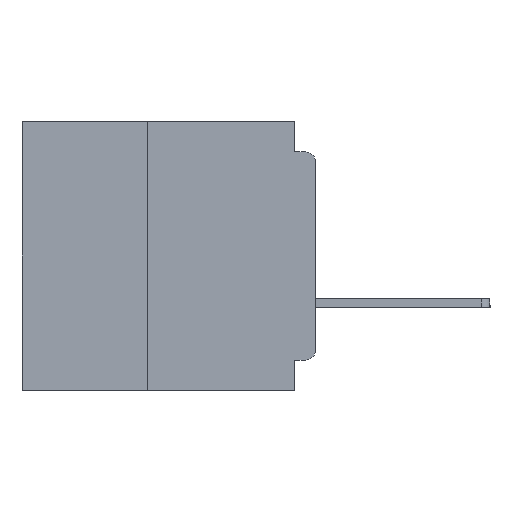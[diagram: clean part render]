
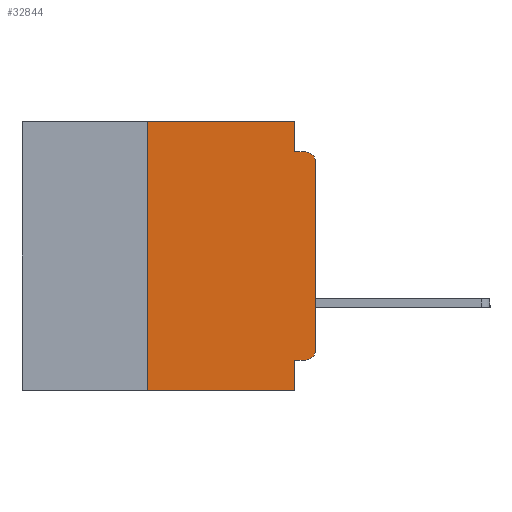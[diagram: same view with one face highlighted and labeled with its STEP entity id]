
A CAD part, left-side view. The second image highlights one B-rep face of the part: STEP entity #32844.
In plain terms, the highlighted planar face has unit normal (-1, 0, 0).
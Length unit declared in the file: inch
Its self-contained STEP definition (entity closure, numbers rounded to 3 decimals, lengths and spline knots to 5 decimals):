
#285 = CARTESIAN_POINT ( 'NONE',  ( 0., 0.031, 0. ) ) ;
#954 = VERTEX_POINT ( 'NONE', #4387 ) ;
#1689 = VERTEX_POINT ( 'NONE', #49540 ) ;
#2049 = AXIS2_PLACEMENT_3D ( 'NONE', #21257, #50289, #25529 ) ;
#2077 = VECTOR ( 'NONE', #4523, 39.37008 ) ;
#2186 = DIRECTION ( 'NONE',  ( 0., 0., 1. ) ) ;
#3131 = AXIS2_PLACEMENT_3D ( 'NONE', #6478, #35747, #10696 ) ;
#3907 = DIRECTION ( 'NONE',  ( 0., 0., 1. ) ) ;
#4387 = CARTESIAN_POINT ( 'NONE',  ( 0., 0.031, 0. ) ) ;
#4523 = DIRECTION ( 'NONE',  ( 0., 0., -1. ) ) ;
#4604 = CARTESIAN_POINT ( 'NONE',  ( 0., 0.031, -0.4 ) ) ;
#5560 = DIRECTION ( 'NONE',  ( 0., -1., 0. ) ) ;
#6478 = CARTESIAN_POINT ( 'NONE',  ( 0., 0.015, -0.06 ) ) ;
#6926 = ORIENTED_EDGE ( 'NONE', *, *, #47745, .F. ) ;
#7359 = EDGE_LOOP ( 'NONE', ( #17656, #30911, #20954, #6926, #18402, #23933, #37663, #18087, #9277, #52777 ) ) ;
#7463 = VERTEX_POINT ( 'NONE', #11105 ) ;
#7567 = DIRECTION ( 'NONE',  ( 1., 0., 0. ) ) ;
#7689 = CARTESIAN_POINT ( 'NONE',  ( 0., 0.437, 0. ) ) ;
#8110 = CARTESIAN_POINT ( 'NONE',  ( 0., 0.437, -0.4 ) ) ;
#9277 = ORIENTED_EDGE ( 'NONE', *, *, #38610, .F. ) ;
#10324 = CARTESIAN_POINT ( 'NONE',  ( 0., 0.031, -0.355 ) ) ;
#10675 = DIRECTION ( 'NONE',  ( 0., 1., 0. ) ) ;
#10696 = DIRECTION ( 'NONE',  ( 0., 0., -1. ) ) ;
#10707 = CARTESIAN_POINT ( 'NONE',  ( 0., 0.031, -0.045 ) ) ;
#11105 = CARTESIAN_POINT ( 'NONE',  ( 0., 0.015, -0.045 ) ) ;
#11180 = CARTESIAN_POINT ( 'NONE',  ( 0., 0.031, -0.4 ) ) ;
#11602 = VECTOR ( 'NONE', #5560, 39.37008 ) ;
#12342 = DIRECTION ( 'NONE',  ( 0., -1., 0. ) ) ;
#12680 = VECTOR ( 'NONE', #3907, 39.37008 ) ;
#13658 = VERTEX_POINT ( 'NONE', #24235 ) ;
#14027 = LINE ( 'NONE', #53820, #12680 ) ;
#17397 = CARTESIAN_POINT ( 'NONE',  ( 0., 0.25, -0.4 ) ) ;
#17582 = VECTOR ( 'NONE', #2186, 39.37008 ) ;
#17656 = ORIENTED_EDGE ( 'NONE', *, *, #22435, .T. ) ;
#18014 = VERTEX_POINT ( 'NONE', #10324 ) ;
#18087 = ORIENTED_EDGE ( 'NONE', *, *, #38323, .F. ) ;
#18402 = ORIENTED_EDGE ( 'NONE', *, *, #29087, .F. ) ;
#18899 = LINE ( 'NONE', #43795, #17582 ) ;
#20417 = VERTEX_POINT ( 'NONE', #11180 ) ;
#20954 = ORIENTED_EDGE ( 'NONE', *, *, #46346, .F. ) ;
#21257 = CARTESIAN_POINT ( 'NONE',  ( 0., 0.015, -0.34 ) ) ;
#21831 = EDGE_CURVE ( 'NONE', #1689, #7463, #37827, .T. ) ;
#22324 = CARTESIAN_POINT ( 'NONE',  ( 0., 0.25, 0. ) ) ;
#22435 = EDGE_CURVE ( 'NONE', #38889, #1689, #18899, .T. ) ;
#22738 = VECTOR ( 'NONE', #10675, 39.37008 ) ;
#22777 = LINE ( 'NONE', #30699, #11602 ) ;
#23933 = ORIENTED_EDGE ( 'NONE', *, *, #40884, .F. ) ;
#24235 = CARTESIAN_POINT ( 'NONE',  ( 0., 0.015, -0.355 ) ) ;
#24778 = VECTOR ( 'NONE', #12342, 39.37008 ) ;
#25529 = DIRECTION ( 'NONE',  ( 0., 0., -1. ) ) ;
#25996 = VERTEX_POINT ( 'NONE', #22324 ) ;
#26074 = VECTOR ( 'NONE', #38063, 39.37008 ) ;
#27151 = CIRCLE ( 'NONE', #2049, 0.015 ) ;
#28562 = EDGE_CURVE ( 'NONE', #45716, #20417, #46804, .T. ) ;
#29087 = EDGE_CURVE ( 'NONE', #25996, #954, #45269, .T. ) ;
#30122 = EDGE_CURVE ( 'NONE', #13658, #38889, #27151, .T. ) ;
#30699 = CARTESIAN_POINT ( 'NONE',  ( 0., 0., -0.045 ) ) ;
#30911 = ORIENTED_EDGE ( 'NONE', *, *, #21831, .T. ) ;
#32457 = CARTESIAN_POINT ( 'NONE',  ( 0., 0.437, 0. ) ) ;
#32638 = PLANE ( 'NONE',  #47627 ) ;
#32844 = ADVANCED_FACE ( 'NONE', ( #38402 ), #32638, .F. ) ;
#33771 = LINE ( 'NONE', #39682, #22738 ) ;
#34236 = VECTOR ( 'NONE', #36920, 39.37008 ) ;
#35487 = LINE ( 'NONE', #285, #2077 ) ;
#35747 = DIRECTION ( 'NONE',  ( -1., 0., 0. ) ) ;
#36804 = DIRECTION ( 'NONE',  ( 0., 0., -1. ) ) ;
#36920 = DIRECTION ( 'NONE',  ( 0., -1., 0. ) ) ;
#37663 = ORIENTED_EDGE ( 'NONE', *, *, #28562, .T. ) ;
#37827 = CIRCLE ( 'NONE', #3131, 0.015 ) ;
#38063 = DIRECTION ( 'NONE',  ( 0., 0., -1. ) ) ;
#38323 = EDGE_CURVE ( 'NONE', #18014, #20417, #39644, .T. ) ;
#38402 = FACE_OUTER_BOUND ( 'NONE', #7359, .T. ) ;
#38610 = EDGE_CURVE ( 'NONE', #13658, #18014, #33771, .T. ) ;
#38889 = VERTEX_POINT ( 'NONE', #42359 ) ;
#39644 = LINE ( 'NONE', #4604, #26074 ) ;
#39682 = CARTESIAN_POINT ( 'NONE',  ( 0., 0., -0.355 ) ) ;
#40884 = EDGE_CURVE ( 'NONE', #45716, #25996, #14027, .T. ) ;
#42359 = CARTESIAN_POINT ( 'NONE',  ( 0., 0., -0.34 ) ) ;
#43072 = VERTEX_POINT ( 'NONE', #10707 ) ;
#43795 = CARTESIAN_POINT ( 'NONE',  ( 0., 0., 0. ) ) ;
#45269 = LINE ( 'NONE', #7689, #34236 ) ;
#45716 = VERTEX_POINT ( 'NONE', #17397 ) ;
#46346 = EDGE_CURVE ( 'NONE', #43072, #7463, #22777, .T. ) ;
#46804 = LINE ( 'NONE', #8110, #24778 ) ;
#47627 = AXIS2_PLACEMENT_3D ( 'NONE', #32457, #7567, #36804 ) ;
#47745 = EDGE_CURVE ( 'NONE', #954, #43072, #35487, .T. ) ;
#49540 = CARTESIAN_POINT ( 'NONE',  ( 0., 0., -0.06 ) ) ;
#50289 = DIRECTION ( 'NONE',  ( -1., 0., 0. ) ) ;
#52777 = ORIENTED_EDGE ( 'NONE', *, *, #30122, .T. ) ;
#53820 = CARTESIAN_POINT ( 'NONE',  ( 0., 0.25, -0.4 ) ) ;
